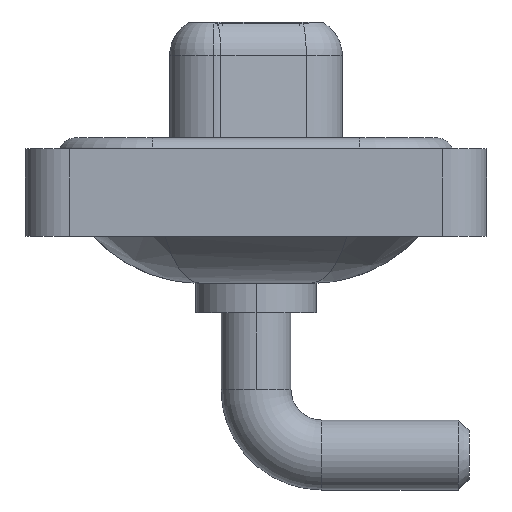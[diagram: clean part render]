
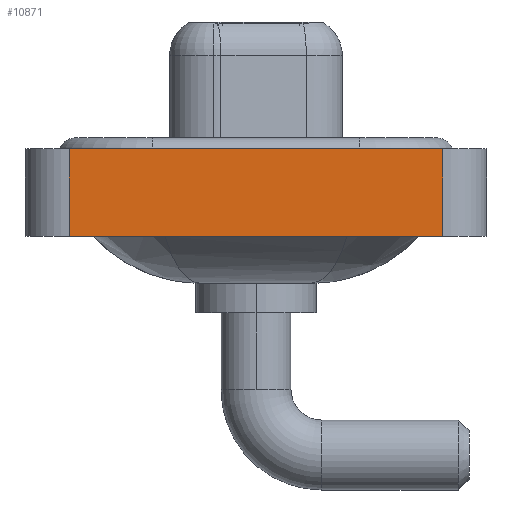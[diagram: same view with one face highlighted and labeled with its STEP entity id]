
A CAD part, left-side view. The second image highlights one B-rep face of the part: STEP entity #10871.
In plain terms, the highlighted planar face has unit normal (-1, 0, 0).
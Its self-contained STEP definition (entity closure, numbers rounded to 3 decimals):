
#89 = DIRECTION ( 'NONE',  ( 0., 0., 1. ) ) ;
#245 = DIRECTION ( 'NONE',  ( 0., 0., 1. ) ) ;
#324 = CARTESIAN_POINT ( 'NONE',  ( -7.25, -8.55, -3.6 ) ) ;
#513 = ORIENTED_EDGE ( 'NONE', *, *, #8959, .T. ) ;
#653 = VERTEX_POINT ( 'NONE', #5836 ) ;
#682 = CARTESIAN_POINT ( 'NONE',  ( -7.25, 8.55, 0.4 ) ) ;
#795 = EDGE_CURVE ( 'NONE', #4856, #653, #4814, .T. ) ;
#924 = LINE ( 'NONE', #11608, #12378 ) ;
#1212 = LINE ( 'NONE', #14749, #9776 ) ;
#1659 = VECTOR ( 'NONE', #3620, 1000. ) ;
#1685 = FACE_OUTER_BOUND ( 'NONE', #8908, .T. ) ;
#1794 = CARTESIAN_POINT ( 'NONE',  ( -7.25, -8.55, 0.4 ) ) ;
#2806 = VERTEX_POINT ( 'NONE', #682 ) ;
#2951 = VECTOR ( 'NONE', #6852, 1000. ) ;
#3620 = DIRECTION ( 'NONE',  ( 0., 0., 1. ) ) ;
#3793 = CARTESIAN_POINT ( 'NONE',  ( -7.25, -8.55, -3.6 ) ) ;
#4814 = LINE ( 'NONE', #9659, #1659 ) ;
#4856 = VERTEX_POINT ( 'NONE', #3793 ) ;
#5532 = DIRECTION ( 'NONE',  ( 0., -1., 0. ) ) ;
#5836 = CARTESIAN_POINT ( 'NONE',  ( -7.25, -8.55, 0.4 ) ) ;
#6441 = ORIENTED_EDGE ( 'NONE', *, *, #8061, .F. ) ;
#6852 = DIRECTION ( 'NONE',  ( 0., -1., 0. ) ) ;
#7616 = PLANE ( 'NONE',  #14090 ) ;
#7805 = LINE ( 'NONE', #1794, #2951 ) ;
#8061 = EDGE_CURVE ( 'NONE', #2806, #653, #7805, .T. ) ;
#8426 = ORIENTED_EDGE ( 'NONE', *, *, #14542, .F. ) ;
#8817 = DIRECTION ( 'NONE',  ( -1., 0., 0. ) ) ;
#8908 = EDGE_LOOP ( 'NONE', ( #13233, #6441, #8426, #513 ) ) ;
#8959 = EDGE_CURVE ( 'NONE', #9379, #4856, #924, .T. ) ;
#9379 = VERTEX_POINT ( 'NONE', #15319 ) ;
#9659 = CARTESIAN_POINT ( 'NONE',  ( -7.25, -8.55, -3.6 ) ) ;
#9776 = VECTOR ( 'NONE', #89, 1000. ) ;
#10871 = ADVANCED_FACE ( 'NONE', ( #1685 ), #7616, .T. ) ;
#11608 = CARTESIAN_POINT ( 'NONE',  ( -7.25, -8.55, -3.6 ) ) ;
#12378 = VECTOR ( 'NONE', #5532, 1000. ) ;
#13233 = ORIENTED_EDGE ( 'NONE', *, *, #795, .T. ) ;
#14090 = AXIS2_PLACEMENT_3D ( 'NONE', #324, #8817, #245 ) ;
#14542 = EDGE_CURVE ( 'NONE', #9379, #2806, #1212, .T. ) ;
#14749 = CARTESIAN_POINT ( 'NONE',  ( -7.25, 8.55, -3.6 ) ) ;
#15319 = CARTESIAN_POINT ( 'NONE',  ( -7.25, 8.55, -3.6 ) ) ;
